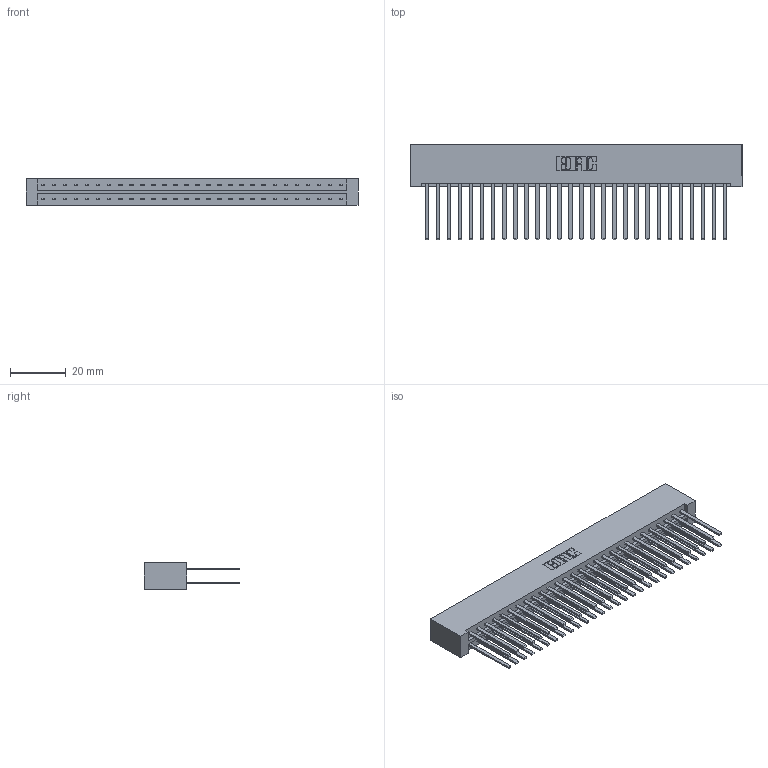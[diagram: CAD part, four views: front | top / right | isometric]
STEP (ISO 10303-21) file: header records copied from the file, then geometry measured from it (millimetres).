
FILE_DESCRIPTION (( 'STEP AP203' ), '1' );
FILE_NAME ('333-056-544-201.STEP', '2018-08-04T05:02:26', ( '' ), ( '' ), 'SwSTEP 2.0', 'SolidWorks 2016', '' );
FILE_SCHEMA (( 'CONFIG_CONTROL_DESIGN' ));
Length unit declared in the file: inch
Products named in the file (3): 333 Part_Lugless; 345-292-001_345-293-144; 333-056-544-201
Assembly tree (57 placements, depth 2):
  333-056-544-201
    333 Part_Lugless
    345-292-001_345-293-144  x56
Bounding box: 119.2 x 34.3 x 9.4 mm (x, y, z)
Volume: 13456.2 mm3; surface area: 18310 mm2
Topology: 57 solids, 57 shells, 2682 faces, 7959 edges, 5230 vertices
Faces by surface type: plane 1858, cylinder 824
Entity records: 19363 total; most frequent: CARTESIAN_POINT 3222, ORIENTED_EDGE 3158, DIRECTION 2767, EDGE_CURVE 1579, LINE 1463, VECTOR 1463, VERTEX_POINT 1050, AXIS2_PLACEMENT_3D 652
